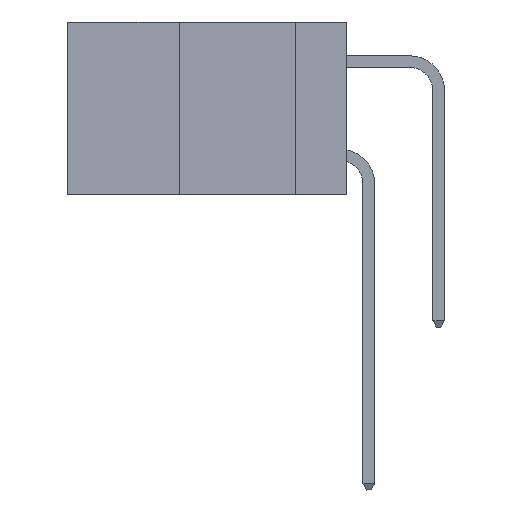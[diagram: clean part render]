
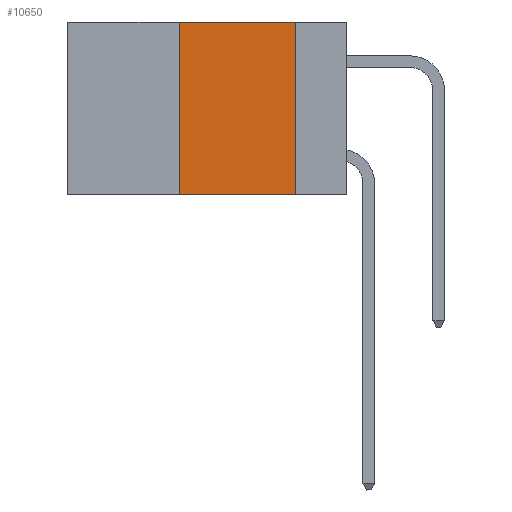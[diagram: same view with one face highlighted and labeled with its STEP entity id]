
A CAD part, left-side view. The second image highlights one B-rep face of the part: STEP entity #10650.
In plain terms, the highlighted planar face has unit normal (-1, 0, 0).
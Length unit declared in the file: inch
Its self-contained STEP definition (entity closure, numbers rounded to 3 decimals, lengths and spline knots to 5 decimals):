
#331 = CARTESIAN_POINT ( 'NONE',  ( 0., 0.6, -0.37 ) ) ;
#2149 = CARTESIAN_POINT ( 'NONE',  ( 0., 0.11, -0.37 ) ) ;
#2409 = EDGE_CURVE ( 'NONE', #16841, #29297, #9338, .T. ) ;
#3380 = CARTESIAN_POINT ( 'NONE',  ( 0., 0.6, 0. ) ) ;
#4245 = DIRECTION ( 'NONE',  ( 0., 0., -1. ) ) ;
#7229 = EDGE_CURVE ( 'NONE', #34653, #16841, #32926, .T. ) ;
#7254 = CARTESIAN_POINT ( 'NONE',  ( 0., 0.11, 0. ) ) ;
#7420 = DIRECTION ( 'NONE',  ( 1., 0., 0. ) ) ;
#9338 = LINE ( 'NONE', #3380, #12289 ) ;
#10650 = ADVANCED_FACE ( 'NONE', ( #36340 ), #23046, .F. ) ;
#10937 = LINE ( 'NONE', #7254, #18351 ) ;
#12289 = VECTOR ( 'NONE', #38050, 39.37008 ) ;
#13625 = ORIENTED_EDGE ( 'NONE', *, *, #7229, .F. ) ;
#16841 = VERTEX_POINT ( 'NONE', #38047 ) ;
#16968 = DIRECTION ( 'NONE',  ( 0., 0., -1. ) ) ;
#18351 = VECTOR ( 'NONE', #16968, 39.37008 ) ;
#22929 = ORIENTED_EDGE ( 'NONE', *, *, #35197, .F. ) ;
#23046 = PLANE ( 'NONE',  #33202 ) ;
#24208 = CARTESIAN_POINT ( 'NONE',  ( 0., 0.36, 0. ) ) ;
#26208 = CARTESIAN_POINT ( 'NONE',  ( 0., 0.6, 0. ) ) ;
#26792 = CARTESIAN_POINT ( 'NONE',  ( 0., 0.11, 0. ) ) ;
#27633 = EDGE_LOOP ( 'NONE', ( #22929, #31279, #13625, #32236 ) ) ;
#29297 = VERTEX_POINT ( 'NONE', #26792 ) ;
#29492 = VECTOR ( 'NONE', #36291, 39.37008 ) ;
#31279 = ORIENTED_EDGE ( 'NONE', *, *, #2409, .F. ) ;
#32021 = VECTOR ( 'NONE', #32033, 39.37008 ) ;
#32033 = DIRECTION ( 'NONE',  ( 0., -1., 0. ) ) ;
#32236 = ORIENTED_EDGE ( 'NONE', *, *, #35756, .T. ) ;
#32926 = LINE ( 'NONE', #24208, #29492 ) ;
#33002 = LINE ( 'NONE', #331, #32021 ) ;
#33202 = AXIS2_PLACEMENT_3D ( 'NONE', #26208, #7420, #4245 ) ;
#34653 = VERTEX_POINT ( 'NONE', #38815 ) ;
#35197 = EDGE_CURVE ( 'NONE', #29297, #35462, #10937, .T. ) ;
#35462 = VERTEX_POINT ( 'NONE', #2149 ) ;
#35756 = EDGE_CURVE ( 'NONE', #34653, #35462, #33002, .T. ) ;
#36291 = DIRECTION ( 'NONE',  ( 0., 0., 1. ) ) ;
#36340 = FACE_OUTER_BOUND ( 'NONE', #27633, .T. ) ;
#38047 = CARTESIAN_POINT ( 'NONE',  ( 0., 0.36, 0. ) ) ;
#38050 = DIRECTION ( 'NONE',  ( 0., -1., 0. ) ) ;
#38815 = CARTESIAN_POINT ( 'NONE',  ( 0., 0.36, -0.37 ) ) ;
